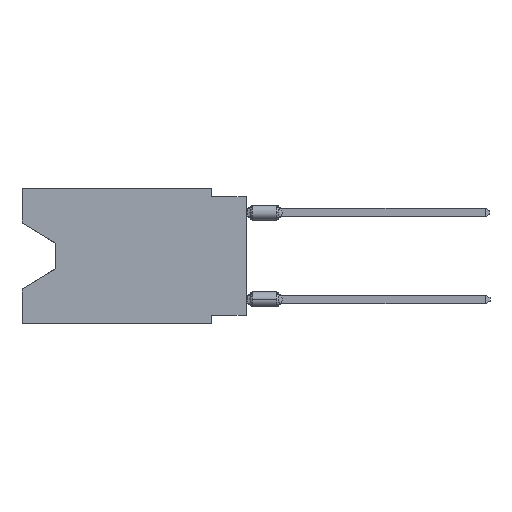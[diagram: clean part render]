
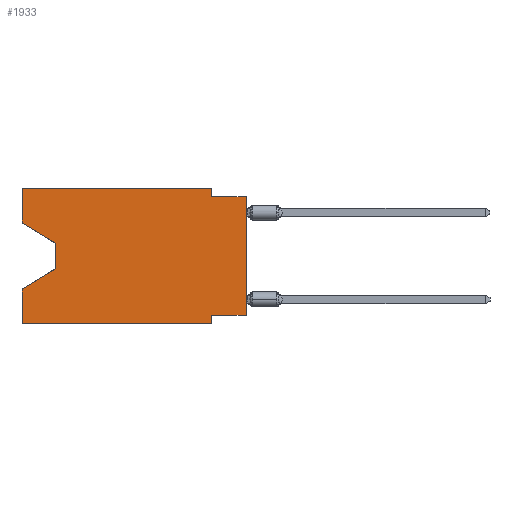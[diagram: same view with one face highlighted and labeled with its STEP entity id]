
A CAD part, left-side view. The second image highlights one B-rep face of the part: STEP entity #1933.
In plain terms, the highlighted planar face has unit normal (-1, 0, 0).
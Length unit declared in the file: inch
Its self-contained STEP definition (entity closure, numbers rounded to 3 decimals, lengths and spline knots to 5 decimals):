
#1145 = ORIENTED_EDGE ( 'NONE', *, *, #56150, .T. ) ;
#1933 = ADVANCED_FACE ( 'NONE', ( #48206 ), #43612, .F. ) ;
#2581 = CARTESIAN_POINT ( 'NONE',  ( 0., 0.1, -0.025 ) ) ;
#3230 = DIRECTION ( 'NONE',  ( 0., 0., -1. ) ) ;
#4321 = VECTOR ( 'NONE', #48110, 39.37008 ) ;
#4513 = VECTOR ( 'NONE', #34017, 39.37008 ) ;
#5165 = CARTESIAN_POINT ( 'NONE',  ( 0., 0.55, -0.232 ) ) ;
#6093 = EDGE_CURVE ( 'NONE', #58447, #46934, #29086, .T. ) ;
#6777 = VECTOR ( 'NONE', #32252, 39.37008 ) ;
#9350 = CARTESIAN_POINT ( 'NONE',  ( 0., 0.1, 0. ) ) ;
#9585 = LINE ( 'NONE', #29613, #37629 ) ;
#10203 = ORIENTED_EDGE ( 'NONE', *, *, #43096, .F. ) ;
#10272 = VECTOR ( 'NONE', #49138, 39.37008 ) ;
#11526 = VECTOR ( 'NONE', #39670, 39.37008 ) ;
#12159 = CARTESIAN_POINT ( 'NONE',  ( 0., 0., -0.365 ) ) ;
#13057 = VECTOR ( 'NONE', #56803, 39.37008 ) ;
#13412 = EDGE_CURVE ( 'NONE', #36505, #23881, #60422, .T. ) ;
#13969 = CARTESIAN_POINT ( 'NONE',  ( 0., 0.645, 0. ) ) ;
#14312 = EDGE_CURVE ( 'NONE', #36667, #59722, #27976, .T. ) ;
#14664 = EDGE_CURVE ( 'NONE', #58447, #23881, #46324, .T. ) ;
#15926 = ORIENTED_EDGE ( 'NONE', *, *, #40174, .T. ) ;
#16405 = CARTESIAN_POINT ( 'NONE',  ( 0., 0.645, -0.39 ) ) ;
#17540 = LINE ( 'NONE', #37595, #4321 ) ;
#17643 = CARTESIAN_POINT ( 'NONE',  ( 0., 0., -0.025 ) ) ;
#17965 = CARTESIAN_POINT ( 'NONE',  ( 0., 0.645, 0. ) ) ;
#19937 = LINE ( 'NONE', #33765, #11526 ) ;
#20276 = VECTOR ( 'NONE', #43954, 39.37008 ) ;
#21489 = CARTESIAN_POINT ( 'NONE',  ( 0., 0.1, -0.39 ) ) ;
#21491 = ORIENTED_EDGE ( 'NONE', *, *, #6093, .F. ) ;
#22192 = VECTOR ( 'NONE', #49631, 39.37008 ) ;
#22378 = CARTESIAN_POINT ( 'NONE',  ( 0., 0.55, -0.158 ) ) ;
#23081 = ORIENTED_EDGE ( 'NONE', *, *, #40971, .F. ) ;
#23256 = EDGE_CURVE ( 'NONE', #60909, #36505, #19937, .T. ) ;
#23881 = VERTEX_POINT ( 'NONE', #21489 ) ;
#23950 = EDGE_CURVE ( 'NONE', #45056, #26381, #17540, .T. ) ;
#24097 = CARTESIAN_POINT ( 'NONE',  ( 0., 0.1, -0.365 ) ) ;
#25424 = ORIENTED_EDGE ( 'NONE', *, *, #23950, .F. ) ;
#25716 = EDGE_CURVE ( 'NONE', #26381, #30533, #9585, .T. ) ;
#26348 = VECTOR ( 'NONE', #29957, 39.37008 ) ;
#26381 = VERTEX_POINT ( 'NONE', #2581 ) ;
#26556 = ORIENTED_EDGE ( 'NONE', *, *, #14664, .T. ) ;
#27976 = LINE ( 'NONE', #22378, #6777 ) ;
#28171 = CARTESIAN_POINT ( 'NONE',  ( 0., 0.645, -0.10025 ) ) ;
#28978 = CARTESIAN_POINT ( 'NONE',  ( 0., 0., 0. ) ) ;
#29086 = LINE ( 'NONE', #54050, #10272 ) ;
#29555 = LINE ( 'NONE', #48955, #60160 ) ;
#29613 = CARTESIAN_POINT ( 'NONE',  ( 0., 0., -0.025 ) ) ;
#29957 = DIRECTION ( 'NONE',  ( 0., 0., 1. ) ) ;
#29975 = VERTEX_POINT ( 'NONE', #56498 ) ;
#30533 = VERTEX_POINT ( 'NONE', #17643 ) ;
#30688 = EDGE_CURVE ( 'NONE', #59722, #46934, #39002, .T. ) ;
#30836 = ORIENTED_EDGE ( 'NONE', *, *, #13412, .F. ) ;
#32252 = DIRECTION ( 'NONE',  ( 0., 0., -1. ) ) ;
#32388 = CARTESIAN_POINT ( 'NONE',  ( 0., 0.645, -0.39 ) ) ;
#32869 = CARTESIAN_POINT ( 'NONE',  ( 0., 0.645, -0.28975 ) ) ;
#33765 = CARTESIAN_POINT ( 'NONE',  ( 0., 0., -0.365 ) ) ;
#34017 = DIRECTION ( 'NONE',  ( 0., -1., 0. ) ) ;
#35588 = CARTESIAN_POINT ( 'NONE',  ( 0., 0.55, -0.158 ) ) ;
#36505 = VERTEX_POINT ( 'NONE', #24097 ) ;
#36667 = VERTEX_POINT ( 'NONE', #35588 ) ;
#36844 = ORIENTED_EDGE ( 'NONE', *, *, #25716, .F. ) ;
#37595 = CARTESIAN_POINT ( 'NONE',  ( 0., 0.1, 0. ) ) ;
#37629 = VECTOR ( 'NONE', #37939, 39.37008 ) ;
#37939 = DIRECTION ( 'NONE',  ( 0., -1., 0. ) ) ;
#39002 = LINE ( 'NONE', #5165, #55488 ) ;
#39369 = AXIS2_PLACEMENT_3D ( 'NONE', #17965, #48533, #3230 ) ;
#39670 = DIRECTION ( 'NONE',  ( 0., 1., 0. ) ) ;
#39937 = VERTEX_POINT ( 'NONE', #60696 ) ;
#40174 = EDGE_CURVE ( 'NONE', #29975, #36667, #48544, .T. ) ;
#40971 = EDGE_CURVE ( 'NONE', #29975, #39937, #29555, .T. ) ;
#41493 = EDGE_LOOP ( 'NONE', ( #15926, #57557, #61089, #21491, #26556, #30836, #60094, #1145, #36844, #25424, #10203, #23081 ) ) ;
#42955 = CARTESIAN_POINT ( 'NONE',  ( 0., 0.55, -0.232 ) ) ;
#43096 = EDGE_CURVE ( 'NONE', #39937, #45056, #58975, .T. ) ;
#43612 = PLANE ( 'NONE',  #39369 ) ;
#43954 = DIRECTION ( 'NONE',  ( 0., -0.855, -0.519 ) ) ;
#44262 = DIRECTION ( 'NONE',  ( 0., 0.855, -0.519 ) ) ;
#45056 = VERTEX_POINT ( 'NONE', #9350 ) ;
#45997 = CARTESIAN_POINT ( 'NONE',  ( 0., 0.1, -0.39 ) ) ;
#46324 = LINE ( 'NONE', #16405, #13057 ) ;
#46934 = VERTEX_POINT ( 'NONE', #32869 ) ;
#48110 = DIRECTION ( 'NONE',  ( 0., 0., -1. ) ) ;
#48206 = FACE_OUTER_BOUND ( 'NONE', #41493, .T. ) ;
#48533 = DIRECTION ( 'NONE',  ( 1., 0., 0. ) ) ;
#48544 = LINE ( 'NONE', #28171, #20276 ) ;
#48955 = CARTESIAN_POINT ( 'NONE',  ( 0., 0.645, 0. ) ) ;
#49138 = DIRECTION ( 'NONE',  ( 0., 0., 1. ) ) ;
#49631 = DIRECTION ( 'NONE',  ( 0., 0., -1. ) ) ;
#54050 = CARTESIAN_POINT ( 'NONE',  ( 0., 0.645, 0. ) ) ;
#55488 = VECTOR ( 'NONE', #44262, 39.37008 ) ;
#56150 = EDGE_CURVE ( 'NONE', #60909, #30533, #64727, .T. ) ;
#56498 = CARTESIAN_POINT ( 'NONE',  ( 0., 0.645, -0.10025 ) ) ;
#56803 = DIRECTION ( 'NONE',  ( 0., -1., 0. ) ) ;
#57557 = ORIENTED_EDGE ( 'NONE', *, *, #14312, .T. ) ;
#58447 = VERTEX_POINT ( 'NONE', #32388 ) ;
#58464 = DIRECTION ( 'NONE',  ( 0., 0., 1. ) ) ;
#58975 = LINE ( 'NONE', #13969, #4513 ) ;
#59722 = VERTEX_POINT ( 'NONE', #42955 ) ;
#60094 = ORIENTED_EDGE ( 'NONE', *, *, #23256, .F. ) ;
#60160 = VECTOR ( 'NONE', #58464, 39.37008 ) ;
#60422 = LINE ( 'NONE', #45997, #22192 ) ;
#60696 = CARTESIAN_POINT ( 'NONE',  ( 0., 0.645, 0. ) ) ;
#60909 = VERTEX_POINT ( 'NONE', #12159 ) ;
#61089 = ORIENTED_EDGE ( 'NONE', *, *, #30688, .T. ) ;
#64727 = LINE ( 'NONE', #28978, #26348 ) ;
